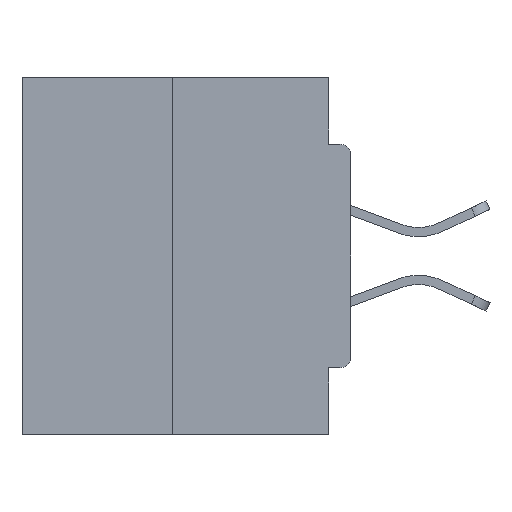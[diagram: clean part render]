
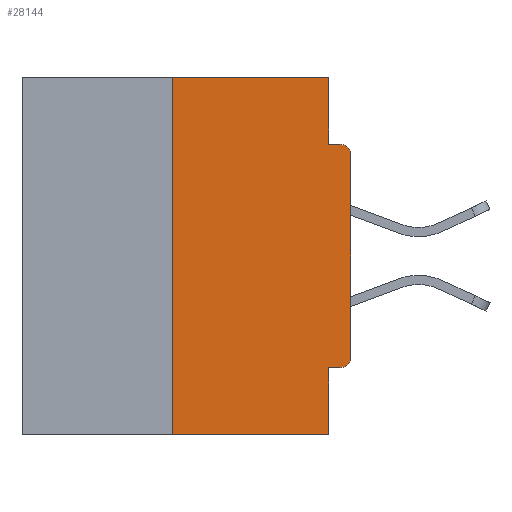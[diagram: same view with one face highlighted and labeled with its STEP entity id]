
A CAD part, left-side view. The second image highlights one B-rep face of the part: STEP entity #28144.
In plain terms, the highlighted planar face has unit normal (-1, 0, 0).
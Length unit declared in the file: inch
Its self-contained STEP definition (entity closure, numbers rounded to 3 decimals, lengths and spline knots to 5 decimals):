
#743 = CIRCLE ( 'NONE', #35567, 0.015 ) ;
#1228 = VERTEX_POINT ( 'NONE', #9385 ) ;
#1332 = CARTESIAN_POINT ( 'NONE',  ( 0., 0., 0. ) ) ;
#1476 = LINE ( 'NONE', #32705, #11391 ) ;
#2512 = ORIENTED_EDGE ( 'NONE', *, *, #11684, .T. ) ;
#2649 = EDGE_CURVE ( 'NONE', #10841, #8415, #5740, .T. ) ;
#2776 = DIRECTION ( 'NONE',  ( 0., 0., -1. ) ) ;
#3206 = LINE ( 'NONE', #14297, #23840 ) ;
#3281 = EDGE_LOOP ( 'NONE', ( #31344, #8376, #21773, #23473, #31240, #15894, #2512, #18310, #29277, #24856 ) ) ;
#3527 = DIRECTION ( 'NONE',  ( 0., 0., -1. ) ) ;
#3638 = VERTEX_POINT ( 'NONE', #30055 ) ;
#3647 = LINE ( 'NONE', #12174, #18713 ) ;
#4254 = CARTESIAN_POINT ( 'NONE',  ( 0., 0.46, 0. ) ) ;
#4854 = CARTESIAN_POINT ( 'NONE',  ( 0., 0., -0.4065 ) ) ;
#4898 = VERTEX_POINT ( 'NONE', #23659 ) ;
#5740 = CIRCLE ( 'NONE', #30551, 0.015 ) ;
#6703 = VERTEX_POINT ( 'NONE', #13286 ) ;
#7394 = FACE_OUTER_BOUND ( 'NONE', #3281, .T. ) ;
#8376 = ORIENTED_EDGE ( 'NONE', *, *, #15336, .F. ) ;
#8415 = VERTEX_POINT ( 'NONE', #21900 ) ;
#9373 = EDGE_CURVE ( 'NONE', #1228, #23330, #11766, .T. ) ;
#9385 = CARTESIAN_POINT ( 'NONE',  ( 0., 0.031, -0.4065 ) ) ;
#9983 = CARTESIAN_POINT ( 'NONE',  ( 0., 0.46, -0.5 ) ) ;
#10364 = CARTESIAN_POINT ( 'NONE',  ( 0., 0.031, -0.5 ) ) ;
#10399 = CARTESIAN_POINT ( 'NONE',  ( 0., 0.031, -0.0935 ) ) ;
#10718 = VERTEX_POINT ( 'NONE', #25710 ) ;
#10841 = VERTEX_POINT ( 'NONE', #11091 ) ;
#11091 = CARTESIAN_POINT ( 'NONE',  ( 0., 0., -0.1085 ) ) ;
#11391 = VECTOR ( 'NONE', #27152, 39.37008 ) ;
#11684 = EDGE_CURVE ( 'NONE', #4898, #10841, #32385, .T. ) ;
#11766 = LINE ( 'NONE', #14745, #15550 ) ;
#12046 = LINE ( 'NONE', #9983, #26031 ) ;
#12141 = DIRECTION ( 'NONE',  ( -1., 0., 0. ) ) ;
#12174 = CARTESIAN_POINT ( 'NONE',  ( 0., 0.46, 0. ) ) ;
#12404 = DIRECTION ( 'NONE',  ( 0., -1., 0. ) ) ;
#12537 = VERTEX_POINT ( 'NONE', #10399 ) ;
#12804 = DIRECTION ( 'NONE',  ( 0., 0., 1. ) ) ;
#12953 = EDGE_CURVE ( 'NONE', #6703, #4898, #743, .T. ) ;
#13195 = DIRECTION ( 'NONE',  ( 0., 1., 0. ) ) ;
#13286 = CARTESIAN_POINT ( 'NONE',  ( 0., 0.015, -0.4065 ) ) ;
#14232 = VERTEX_POINT ( 'NONE', #15096 ) ;
#14297 = CARTESIAN_POINT ( 'NONE',  ( 0., 0., -0.0935 ) ) ;
#14463 = CARTESIAN_POINT ( 'NONE',  ( 0., 0.015, -0.3915 ) ) ;
#14745 = CARTESIAN_POINT ( 'NONE',  ( 0., 0.031, -0.5 ) ) ;
#14823 = DIRECTION ( 'NONE',  ( -1., 0., 0. ) ) ;
#15096 = CARTESIAN_POINT ( 'NONE',  ( 0., 0.031, 0. ) ) ;
#15336 = EDGE_CURVE ( 'NONE', #3638, #10718, #1476, .T. ) ;
#15550 = VECTOR ( 'NONE', #34318, 39.37008 ) ;
#15894 = ORIENTED_EDGE ( 'NONE', *, *, #12953, .T. ) ;
#15901 = EDGE_CURVE ( 'NONE', #12537, #8415, #3206, .T. ) ;
#15991 = AXIS2_PLACEMENT_3D ( 'NONE', #4254, #32723, #18694 ) ;
#16720 = VECTOR ( 'NONE', #13195, 39.37008 ) ;
#17306 = CARTESIAN_POINT ( 'NONE',  ( 0., 0.015, -0.1085 ) ) ;
#18310 = ORIENTED_EDGE ( 'NONE', *, *, #2649, .T. ) ;
#18694 = DIRECTION ( 'NONE',  ( 0., 0., -1. ) ) ;
#18713 = VECTOR ( 'NONE', #23445, 39.37008 ) ;
#21764 = EDGE_CURVE ( 'NONE', #14232, #12537, #33641, .T. ) ;
#21773 = ORIENTED_EDGE ( 'NONE', *, *, #28927, .T. ) ;
#21900 = CARTESIAN_POINT ( 'NONE',  ( 0., 0.015, -0.0935 ) ) ;
#22058 = LINE ( 'NONE', #4854, #16720 ) ;
#22335 = VECTOR ( 'NONE', #2776, 39.37008 ) ;
#23330 = VERTEX_POINT ( 'NONE', #10364 ) ;
#23445 = DIRECTION ( 'NONE',  ( 0., -1., 0. ) ) ;
#23473 = ORIENTED_EDGE ( 'NONE', *, *, #9373, .F. ) ;
#23659 = CARTESIAN_POINT ( 'NONE',  ( 0., 0., -0.3915 ) ) ;
#23840 = VECTOR ( 'NONE', #25568, 39.37008 ) ;
#23957 = VECTOR ( 'NONE', #12804, 39.37008 ) ;
#24856 = ORIENTED_EDGE ( 'NONE', *, *, #21764, .F. ) ;
#25568 = DIRECTION ( 'NONE',  ( 0., -1., 0. ) ) ;
#25710 = CARTESIAN_POINT ( 'NONE',  ( 0., 0.25, 0. ) ) ;
#25822 = DIRECTION ( 'NONE',  ( 0., 0., -1. ) ) ;
#26031 = VECTOR ( 'NONE', #12404, 39.37008 ) ;
#27152 = DIRECTION ( 'NONE',  ( 0., 0., 1. ) ) ;
#28144 = ADVANCED_FACE ( 'NONE', ( #7394 ), #29761, .F. ) ;
#28927 = EDGE_CURVE ( 'NONE', #3638, #23330, #12046, .T. ) ;
#29277 = ORIENTED_EDGE ( 'NONE', *, *, #15901, .F. ) ;
#29761 = PLANE ( 'NONE',  #15991 ) ;
#30055 = CARTESIAN_POINT ( 'NONE',  ( 0., 0.25, -0.5 ) ) ;
#30551 = AXIS2_PLACEMENT_3D ( 'NONE', #17306, #12141, #25822 ) ;
#30863 = CARTESIAN_POINT ( 'NONE',  ( 0., 0.031, 0. ) ) ;
#31240 = ORIENTED_EDGE ( 'NONE', *, *, #32675, .F. ) ;
#31344 = ORIENTED_EDGE ( 'NONE', *, *, #36430, .F. ) ;
#32385 = LINE ( 'NONE', #1332, #23957 ) ;
#32675 = EDGE_CURVE ( 'NONE', #6703, #1228, #22058, .T. ) ;
#32705 = CARTESIAN_POINT ( 'NONE',  ( 0., 0.25, 0. ) ) ;
#32723 = DIRECTION ( 'NONE',  ( 1., 0., 0. ) ) ;
#33641 = LINE ( 'NONE', #30863, #22335 ) ;
#34318 = DIRECTION ( 'NONE',  ( 0., 0., -1. ) ) ;
#35567 = AXIS2_PLACEMENT_3D ( 'NONE', #14463, #14823, #3527 ) ;
#36430 = EDGE_CURVE ( 'NONE', #10718, #14232, #3647, .T. ) ;
